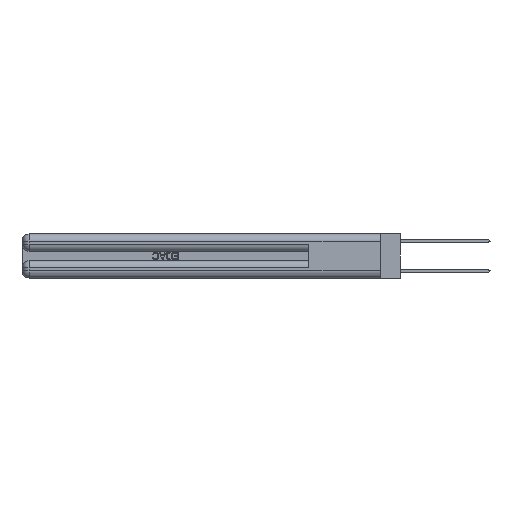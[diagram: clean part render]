
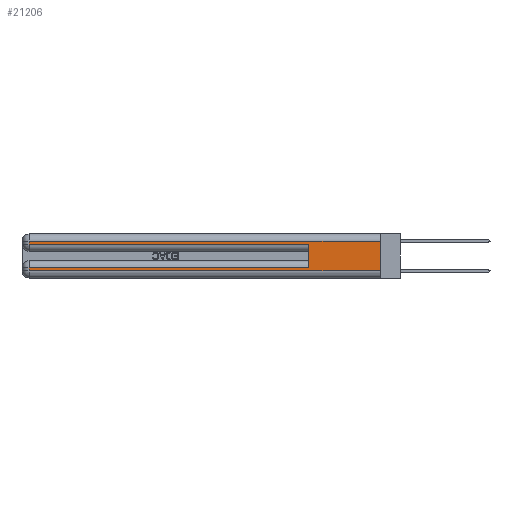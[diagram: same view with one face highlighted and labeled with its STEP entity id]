
A CAD part, left-side view. The second image highlights one B-rep face of the part: STEP entity #21206.
In plain terms, the highlighted planar face has unit normal (-1, 0, 0).
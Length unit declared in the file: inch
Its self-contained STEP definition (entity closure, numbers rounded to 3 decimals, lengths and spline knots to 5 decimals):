
#311 = CARTESIAN_POINT ( 'NONE',  ( 0., 2.94, 0.085 ) ) ;
#490 = VERTEX_POINT ( 'NONE', #5062 ) ;
#704 = ORIENTED_EDGE ( 'NONE', *, *, #11501, .T. ) ;
#878 = DIRECTION ( 'NONE',  ( 0., 0., -1. ) ) ;
#2557 = LINE ( 'NONE', #10184, #21801 ) ;
#3450 = EDGE_LOOP ( 'NONE', ( #3809, #704, #20877, #9954, #11656, #13876, #17514, #4663 ) ) ;
#3736 = VERTEX_POINT ( 'NONE', #7010 ) ;
#3809 = ORIENTED_EDGE ( 'NONE', *, *, #25036, .F. ) ;
#4119 = LINE ( 'NONE', #13413, #24516 ) ;
#4663 = ORIENTED_EDGE ( 'NONE', *, *, #21492, .T. ) ;
#5062 = CARTESIAN_POINT ( 'NONE',  ( 0., 2.94, 0.31 ) ) ;
#5776 = CARTESIAN_POINT ( 'NONE',  ( 0., 2.94, 0.06 ) ) ;
#5897 = VECTOR ( 'NONE', #7103, 39.37008 ) ;
#6053 = DIRECTION ( 'NONE',  ( 0., -1., 0. ) ) ;
#6262 = LINE ( 'NONE', #24536, #9509 ) ;
#6960 = CARTESIAN_POINT ( 'NONE',  ( 0., 2.94, 0.37 ) ) ;
#7010 = CARTESIAN_POINT ( 'NONE',  ( 0., 0.6, 0.085 ) ) ;
#7099 = CARTESIAN_POINT ( 'NONE',  ( 0., 0., 0.06 ) ) ;
#7103 = DIRECTION ( 'NONE',  ( 0., 0., -1. ) ) ;
#7585 = CARTESIAN_POINT ( 'NONE',  ( 0., 0., 0.31 ) ) ;
#7912 = VERTEX_POINT ( 'NONE', #18386 ) ;
#8102 = EDGE_CURVE ( 'NONE', #490, #29596, #26314, .T. ) ;
#8206 = LINE ( 'NONE', #10335, #14702 ) ;
#8328 = EDGE_CURVE ( 'NONE', #19554, #27896, #25509, .T. ) ;
#8568 = CARTESIAN_POINT ( 'NONE',  ( 0., 0., 0.31 ) ) ;
#9509 = VECTOR ( 'NONE', #20240, 39.37008 ) ;
#9773 = EDGE_CURVE ( 'NONE', #29596, #7912, #11364, .T. ) ;
#9954 = ORIENTED_EDGE ( 'NONE', *, *, #9773, .T. ) ;
#10184 = CARTESIAN_POINT ( 'NONE',  ( 0., 0.6, 0.145 ) ) ;
#10335 = CARTESIAN_POINT ( 'NONE',  ( 0., 0., 0.06 ) ) ;
#10810 = AXIS2_PLACEMENT_3D ( 'NONE', #27542, #22951, #20511 ) ;
#11364 = LINE ( 'NONE', #29815, #24613 ) ;
#11501 = EDGE_CURVE ( 'NONE', #25074, #490, #14270, .T. ) ;
#11581 = EDGE_CURVE ( 'NONE', #3736, #7912, #2557, .T. ) ;
#11656 = ORIENTED_EDGE ( 'NONE', *, *, #11581, .F. ) ;
#12614 = CARTESIAN_POINT ( 'NONE',  ( 0., 2.94, 0.37 ) ) ;
#13413 = CARTESIAN_POINT ( 'NONE',  ( 0., 0., 0.085 ) ) ;
#13876 = ORIENTED_EDGE ( 'NONE', *, *, #25104, .T. ) ;
#14270 = LINE ( 'NONE', #7585, #23751 ) ;
#14403 = VERTEX_POINT ( 'NONE', #7099 ) ;
#14628 = VECTOR ( 'NONE', #878, 39.37008 ) ;
#14702 = VECTOR ( 'NONE', #6053, 39.37008 ) ;
#15743 = CARTESIAN_POINT ( 'NONE',  ( 0., 2.94, 0.285 ) ) ;
#17514 = ORIENTED_EDGE ( 'NONE', *, *, #8328, .T. ) ;
#17666 = DIRECTION ( 'NONE',  ( 0., 1., 0. ) ) ;
#18223 = PLANE ( 'NONE',  #10810 ) ;
#18386 = CARTESIAN_POINT ( 'NONE',  ( 0., 0.6, 0.285 ) ) ;
#18817 = DIRECTION ( 'NONE',  ( 0., 1., 0. ) ) ;
#19554 = VERTEX_POINT ( 'NONE', #311 ) ;
#20240 = DIRECTION ( 'NONE',  ( 0., 0., -1. ) ) ;
#20511 = DIRECTION ( 'NONE',  ( 0., 0., -1. ) ) ;
#20877 = ORIENTED_EDGE ( 'NONE', *, *, #8102, .T. ) ;
#21206 = ADVANCED_FACE ( 'NONE', ( #27099 ), #18223, .F. ) ;
#21492 = EDGE_CURVE ( 'NONE', #27896, #14403, #8206, .T. ) ;
#21719 = DIRECTION ( 'NONE',  ( 0., 0., 1. ) ) ;
#21801 = VECTOR ( 'NONE', #21719, 39.37008 ) ;
#22951 = DIRECTION ( 'NONE',  ( 1., 0., 0. ) ) ;
#23751 = VECTOR ( 'NONE', #18817, 39.37008 ) ;
#24516 = VECTOR ( 'NONE', #17666, 39.37008 ) ;
#24536 = CARTESIAN_POINT ( 'NONE',  ( 0., 0., 0.37 ) ) ;
#24613 = VECTOR ( 'NONE', #25663, 39.37008 ) ;
#25036 = EDGE_CURVE ( 'NONE', #25074, #14403, #6262, .T. ) ;
#25074 = VERTEX_POINT ( 'NONE', #8568 ) ;
#25104 = EDGE_CURVE ( 'NONE', #3736, #19554, #4119, .T. ) ;
#25509 = LINE ( 'NONE', #6960, #5897 ) ;
#25663 = DIRECTION ( 'NONE',  ( 0., -1., 0. ) ) ;
#26314 = LINE ( 'NONE', #12614, #14628 ) ;
#27099 = FACE_OUTER_BOUND ( 'NONE', #3450, .T. ) ;
#27542 = CARTESIAN_POINT ( 'NONE',  ( 0., 0., 0.37 ) ) ;
#27896 = VERTEX_POINT ( 'NONE', #5776 ) ;
#29596 = VERTEX_POINT ( 'NONE', #15743 ) ;
#29815 = CARTESIAN_POINT ( 'NONE',  ( 0., 0., 0.285 ) ) ;
